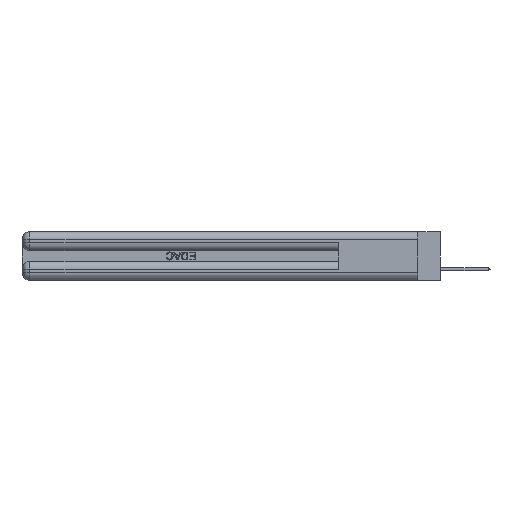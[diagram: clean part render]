
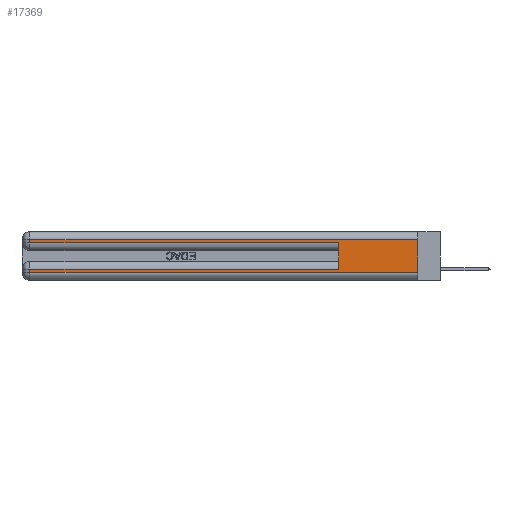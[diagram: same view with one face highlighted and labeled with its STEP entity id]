
A CAD part, left-side view. The second image highlights one B-rep face of the part: STEP entity #17369.
In plain terms, the highlighted planar face has unit normal (-1, 0, 0).
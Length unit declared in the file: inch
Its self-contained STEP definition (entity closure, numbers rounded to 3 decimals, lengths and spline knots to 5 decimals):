
#513 = ORIENTED_EDGE ( 'NONE', *, *, #31578, .T. ) ;
#987 = CARTESIAN_POINT ( 'NONE',  ( 0., 0., 0.06 ) ) ;
#1008 = LINE ( 'NONE', #30345, #49099 ) ;
#1018 = EDGE_LOOP ( 'NONE', ( #21785, #513, #15128, #22062, #4308, #40792, #3080, #9786 ) ) ;
#1194 = LINE ( 'NONE', #37494, #38061 ) ;
#1554 = CARTESIAN_POINT ( 'NONE',  ( 0., 2.94, 0.37 ) ) ;
#1739 = DIRECTION ( 'NONE',  ( 0., 1., 0. ) ) ;
#1809 = CARTESIAN_POINT ( 'NONE',  ( 0., 0., 0.285 ) ) ;
#1881 = EDGE_CURVE ( 'NONE', #7491, #3489, #29297, .T. ) ;
#2205 = VECTOR ( 'NONE', #34582, 39.37008 ) ;
#3080 = ORIENTED_EDGE ( 'NONE', *, *, #47164, .T. ) ;
#3489 = VERTEX_POINT ( 'NONE', #11660 ) ;
#3654 = CARTESIAN_POINT ( 'NONE',  ( 0., 2.94, 0.06 ) ) ;
#4308 = ORIENTED_EDGE ( 'NONE', *, *, #20590, .F. ) ;
#6410 = EDGE_CURVE ( 'NONE', #32455, #13324, #38259, .T. ) ;
#7122 = CARTESIAN_POINT ( 'NONE',  ( 0., 0., 0.31 ) ) ;
#7491 = VERTEX_POINT ( 'NONE', #30115 ) ;
#7611 = FACE_OUTER_BOUND ( 'NONE', #1018, .T. ) ;
#7859 = CARTESIAN_POINT ( 'NONE',  ( 0., 0., 0.37 ) ) ;
#9786 = ORIENTED_EDGE ( 'NONE', *, *, #6410, .T. ) ;
#11660 = CARTESIAN_POINT ( 'NONE',  ( 0., 2.94, 0.285 ) ) ;
#12393 = VERTEX_POINT ( 'NONE', #36292 ) ;
#13324 = VERTEX_POINT ( 'NONE', #987 ) ;
#15128 = ORIENTED_EDGE ( 'NONE', *, *, #1881, .T. ) ;
#15836 = LINE ( 'NONE', #29019, #37650 ) ;
#15913 = DIRECTION ( 'NONE',  ( 0., -1., 0. ) ) ;
#16247 = DIRECTION ( 'NONE',  ( 0., -1., 0. ) ) ;
#16353 = VERTEX_POINT ( 'NONE', #7122 ) ;
#17369 = ADVANCED_FACE ( 'NONE', ( #7611 ), #47793, .F. ) ;
#17804 = LINE ( 'NONE', #46273, #2205 ) ;
#17983 = CARTESIAN_POINT ( 'NONE',  ( 0., 0., 0.085 ) ) ;
#19062 = CARTESIAN_POINT ( 'NONE',  ( 0., 0.6, 0.285 ) ) ;
#20590 = EDGE_CURVE ( 'NONE', #47288, #27574, #15836, .T. ) ;
#20935 = CARTESIAN_POINT ( 'NONE',  ( 0., 0., 0.06 ) ) ;
#21610 = AXIS2_PLACEMENT_3D ( 'NONE', #7859, #43090, #51712 ) ;
#21785 = ORIENTED_EDGE ( 'NONE', *, *, #33813, .F. ) ;
#22062 = ORIENTED_EDGE ( 'NONE', *, *, #41518, .T. ) ;
#26367 = VECTOR ( 'NONE', #15913, 39.37008 ) ;
#26541 = VECTOR ( 'NONE', #50687, 39.37008 ) ;
#27574 = VERTEX_POINT ( 'NONE', #19062 ) ;
#29019 = CARTESIAN_POINT ( 'NONE',  ( 0., 0.6, 0.145 ) ) ;
#29297 = LINE ( 'NONE', #1554, #47470 ) ;
#30115 = CARTESIAN_POINT ( 'NONE',  ( 0., 2.94, 0.31 ) ) ;
#30345 = CARTESIAN_POINT ( 'NONE',  ( 0., 0., 0.31 ) ) ;
#31356 = LINE ( 'NONE', #1809, #26367 ) ;
#31578 = EDGE_CURVE ( 'NONE', #16353, #7491, #1008, .T. ) ;
#32455 = VERTEX_POINT ( 'NONE', #3654 ) ;
#33813 = EDGE_CURVE ( 'NONE', #16353, #13324, #17804, .T. ) ;
#33815 = DIRECTION ( 'NONE',  ( 0., 0., -1. ) ) ;
#34582 = DIRECTION ( 'NONE',  ( 0., 0., -1. ) ) ;
#34959 = DIRECTION ( 'NONE',  ( 0., 0., 1. ) ) ;
#36292 = CARTESIAN_POINT ( 'NONE',  ( 0., 2.94, 0.085 ) ) ;
#37494 = CARTESIAN_POINT ( 'NONE',  ( 0., 2.94, 0.37 ) ) ;
#37650 = VECTOR ( 'NONE', #34959, 39.37008 ) ;
#38061 = VECTOR ( 'NONE', #44971, 39.37008 ) ;
#38259 = LINE ( 'NONE', #20935, #50819 ) ;
#38546 = CARTESIAN_POINT ( 'NONE',  ( 0., 0.6, 0.085 ) ) ;
#40792 = ORIENTED_EDGE ( 'NONE', *, *, #50469, .T. ) ;
#41518 = EDGE_CURVE ( 'NONE', #3489, #27574, #31356, .T. ) ;
#43090 = DIRECTION ( 'NONE',  ( 1., 0., 0. ) ) ;
#44971 = DIRECTION ( 'NONE',  ( 0., 0., -1. ) ) ;
#46273 = CARTESIAN_POINT ( 'NONE',  ( 0., 0., 0.37 ) ) ;
#47164 = EDGE_CURVE ( 'NONE', #12393, #32455, #1194, .T. ) ;
#47288 = VERTEX_POINT ( 'NONE', #38546 ) ;
#47470 = VECTOR ( 'NONE', #33815, 39.37008 ) ;
#47793 = PLANE ( 'NONE',  #21610 ) ;
#47800 = LINE ( 'NONE', #17983, #26541 ) ;
#49099 = VECTOR ( 'NONE', #1739, 39.37008 ) ;
#50469 = EDGE_CURVE ( 'NONE', #47288, #12393, #47800, .T. ) ;
#50687 = DIRECTION ( 'NONE',  ( 0., 1., 0. ) ) ;
#50819 = VECTOR ( 'NONE', #16247, 39.37008 ) ;
#51712 = DIRECTION ( 'NONE',  ( 0., 0., -1. ) ) ;
